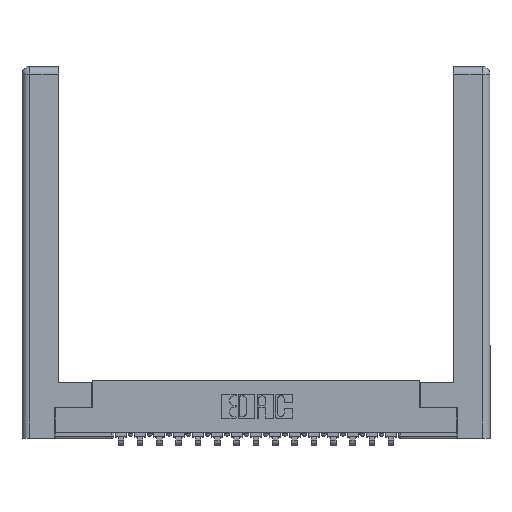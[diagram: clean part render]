
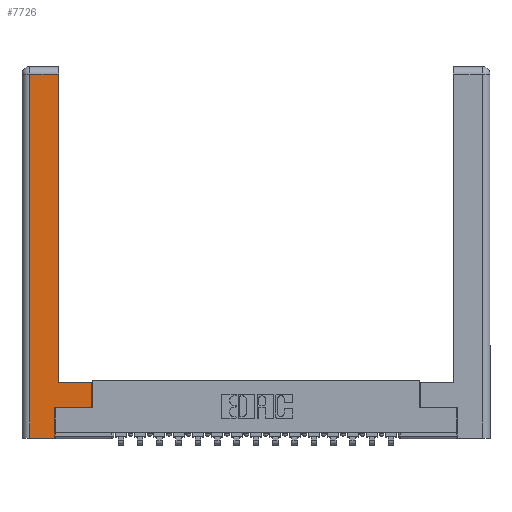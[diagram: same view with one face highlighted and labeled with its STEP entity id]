
A CAD part, top view. The second image highlights one B-rep face of the part: STEP entity #7726.
In plain terms, the highlighted planar face has unit normal (0, 0, 1).
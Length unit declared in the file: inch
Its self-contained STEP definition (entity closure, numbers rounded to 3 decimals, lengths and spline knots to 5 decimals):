
#100 = CARTESIAN_POINT ( 'NONE',  ( 0.565, 0.245, 0. ) ) ;
#504 = ORIENTED_EDGE ( 'NONE', *, *, #12795, .T. ) ;
#769 = CARTESIAN_POINT ( 'NONE',  ( 0.265, 0., 0. ) ) ;
#1185 = PLANE ( 'NONE',  #14646 ) ;
#1453 = VERTEX_POINT ( 'NONE', #11871 ) ;
#1672 = VECTOR ( 'NONE', #9438, 39.37008 ) ;
#2016 = LINE ( 'NONE', #7384, #3901 ) ;
#2610 = EDGE_CURVE ( 'NONE', #9602, #17593, #8846, .T. ) ;
#2983 = CARTESIAN_POINT ( 'NONE',  ( 0.565, 0.45, 0. ) ) ;
#3452 = EDGE_CURVE ( 'NONE', #10713, #19565, #7379, .T. ) ;
#3637 = ORIENTED_EDGE ( 'NONE', *, *, #8576, .T. ) ;
#3901 = VECTOR ( 'NONE', #7316, 39.37008 ) ;
#4003 = LINE ( 'NONE', #100, #1672 ) ;
#4043 = VECTOR ( 'NONE', #15244, 39.37008 ) ;
#4915 = CARTESIAN_POINT ( 'NONE',  ( 0.565, 0.245, 0. ) ) ;
#5727 = CARTESIAN_POINT ( 'NONE',  ( 0.265, 0., 0. ) ) ;
#5740 = ORIENTED_EDGE ( 'NONE', *, *, #12944, .T. ) ;
#5822 = FACE_OUTER_BOUND ( 'NONE', #14176, .T. ) ;
#6474 = VECTOR ( 'NONE', #11995, 39.37008 ) ;
#6499 = CARTESIAN_POINT ( 'NONE',  ( 0.295, 0.45, 0. ) ) ;
#6620 = LINE ( 'NONE', #7739, #4043 ) ;
#7057 = DIRECTION ( 'NONE',  ( 0., 0., -1. ) ) ;
#7316 = DIRECTION ( 'NONE',  ( 0., 1., 0. ) ) ;
#7379 = LINE ( 'NONE', #10971, #14570 ) ;
#7384 = CARTESIAN_POINT ( 'NONE',  ( 0.295, 3., 0. ) ) ;
#7472 = LINE ( 'NONE', #9342, #15634 ) ;
#7726 = ADVANCED_FACE ( 'NONE', ( #5822 ), #1185, .F. ) ;
#7739 = CARTESIAN_POINT ( 'NONE',  ( 0.565, 0.45, 0. ) ) ;
#8111 = VECTOR ( 'NONE', #18705, 39.37008 ) ;
#8576 = EDGE_CURVE ( 'NONE', #17593, #15027, #11702, .T. ) ;
#8776 = CARTESIAN_POINT ( 'NONE',  ( 0., 0., 0. ) ) ;
#8846 = LINE ( 'NONE', #13961, #6474 ) ;
#9219 = ORIENTED_EDGE ( 'NONE', *, *, #19264, .T. ) ;
#9342 = CARTESIAN_POINT ( 'NONE',  ( 0.0615, 2.94, 0. ) ) ;
#9438 = DIRECTION ( 'NONE',  ( 1., 0., 0. ) ) ;
#9589 = ORIENTED_EDGE ( 'NONE', *, *, #15643, .T. ) ;
#9602 = VERTEX_POINT ( 'NONE', #12296 ) ;
#9673 = ORIENTED_EDGE ( 'NONE', *, *, #10805, .T. ) ;
#9909 = ORIENTED_EDGE ( 'NONE', *, *, #3452, .T. ) ;
#10713 = VERTEX_POINT ( 'NONE', #2983 ) ;
#10805 = EDGE_CURVE ( 'NONE', #1453, #12175, #4003, .T. ) ;
#10971 = CARTESIAN_POINT ( 'NONE',  ( 0.295, 0.45, 0. ) ) ;
#11291 = DIRECTION ( 'NONE',  ( 0., 1., 0. ) ) ;
#11702 = LINE ( 'NONE', #769, #8111 ) ;
#11871 = CARTESIAN_POINT ( 'NONE',  ( 0.265, 0.245, 0. ) ) ;
#11995 = DIRECTION ( 'NONE',  ( 0., -1., 0. ) ) ;
#12175 = VERTEX_POINT ( 'NONE', #4915 ) ;
#12296 = CARTESIAN_POINT ( 'NONE',  ( 0.0615, 2.94, 0. ) ) ;
#12702 = CARTESIAN_POINT ( 'NONE',  ( 0.0615, 0., 0. ) ) ;
#12795 = EDGE_CURVE ( 'NONE', #13833, #9602, #7472, .T. ) ;
#12944 = EDGE_CURVE ( 'NONE', #15027, #1453, #14429, .T. ) ;
#13833 = VERTEX_POINT ( 'NONE', #16274 ) ;
#13961 = CARTESIAN_POINT ( 'NONE',  ( 0.0615, 0., 0. ) ) ;
#14171 = CARTESIAN_POINT ( 'NONE',  ( 0.265, 0.245, 0. ) ) ;
#14176 = EDGE_LOOP ( 'NONE', ( #9219, #504, #14530, #3637, #5740, #9673, #9589, #9909 ) ) ;
#14429 = LINE ( 'NONE', #14171, #15147 ) ;
#14530 = ORIENTED_EDGE ( 'NONE', *, *, #2610, .T. ) ;
#14570 = VECTOR ( 'NONE', #17122, 39.37008 ) ;
#14646 = AXIS2_PLACEMENT_3D ( 'NONE', #8776, #7057, #14818 ) ;
#14818 = DIRECTION ( 'NONE',  ( -1., 0., 0. ) ) ;
#15027 = VERTEX_POINT ( 'NONE', #5727 ) ;
#15147 = VECTOR ( 'NONE', #11291, 39.37008 ) ;
#15244 = DIRECTION ( 'NONE',  ( 0., 1., 0. ) ) ;
#15634 = VECTOR ( 'NONE', #16838, 39.37008 ) ;
#15643 = EDGE_CURVE ( 'NONE', #12175, #10713, #6620, .T. ) ;
#16274 = CARTESIAN_POINT ( 'NONE',  ( 0.295, 2.94, 0. ) ) ;
#16838 = DIRECTION ( 'NONE',  ( -1., 0., 0. ) ) ;
#17122 = DIRECTION ( 'NONE',  ( -1., 0., 0. ) ) ;
#17593 = VERTEX_POINT ( 'NONE', #12702 ) ;
#18705 = DIRECTION ( 'NONE',  ( 1., 0., 0. ) ) ;
#19264 = EDGE_CURVE ( 'NONE', #19565, #13833, #2016, .T. ) ;
#19565 = VERTEX_POINT ( 'NONE', #6499 ) ;
